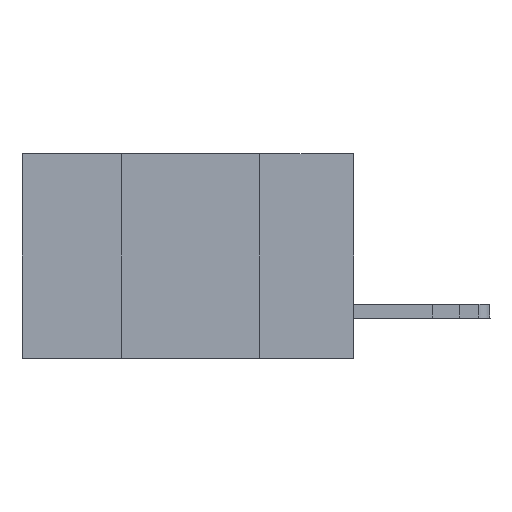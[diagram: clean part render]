
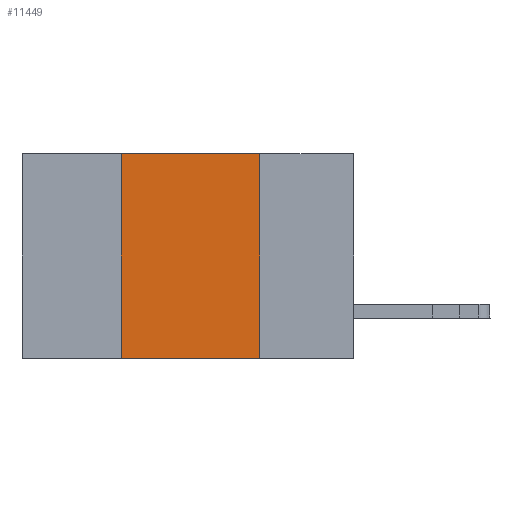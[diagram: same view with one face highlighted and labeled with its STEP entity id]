
A CAD part, left-side view. The second image highlights one B-rep face of the part: STEP entity #11449.
In plain terms, the highlighted planar face has unit normal (-1, 0, 0).
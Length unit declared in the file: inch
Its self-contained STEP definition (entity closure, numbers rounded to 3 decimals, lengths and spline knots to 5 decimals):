
#353 = CARTESIAN_POINT ( 'NONE',  ( 0., 0.42, 0. ) ) ;
#633 = ORIENTED_EDGE ( 'NONE', *, *, #11389, .F. ) ;
#1819 = ORIENTED_EDGE ( 'NONE', *, *, #3543, .F. ) ;
#2001 = VECTOR ( 'NONE', #17645, 39.37008 ) ;
#2810 = CARTESIAN_POINT ( 'NONE',  ( 0., 0.17, 0. ) ) ;
#3543 = EDGE_CURVE ( 'NONE', #6142, #19580, #6987, .T. ) ;
#4345 = ORIENTED_EDGE ( 'NONE', *, *, #11777, .T. ) ;
#4548 = DIRECTION ( 'NONE',  ( 0., -1., 0. ) ) ;
#4571 = EDGE_LOOP ( 'NONE', ( #10133, #633, #1819, #4345 ) ) ;
#5294 = CARTESIAN_POINT ( 'NONE',  ( 0., 0.6, -0.37 ) ) ;
#6142 = VERTEX_POINT ( 'NONE', #9474 ) ;
#6627 = DIRECTION ( 'NONE',  ( 1., 0., 0. ) ) ;
#6987 = LINE ( 'NONE', #353, #10831 ) ;
#8468 = CARTESIAN_POINT ( 'NONE',  ( 0., 0.42, 0. ) ) ;
#8620 = VECTOR ( 'NONE', #10720, 39.37008 ) ;
#9474 = CARTESIAN_POINT ( 'NONE',  ( 0., 0.42, -0.37 ) ) ;
#9942 = LINE ( 'NONE', #19896, #14551 ) ;
#10050 = VERTEX_POINT ( 'NONE', #18899 ) ;
#10133 = ORIENTED_EDGE ( 'NONE', *, *, #16684, .F. ) ;
#10710 = DIRECTION ( 'NONE',  ( 0., 0., 1. ) ) ;
#10720 = DIRECTION ( 'NONE',  ( 0., 0., -1. ) ) ;
#10831 = VECTOR ( 'NONE', #10710, 39.37008 ) ;
#11389 = EDGE_CURVE ( 'NONE', #19580, #10050, #9942, .T. ) ;
#11449 = ADVANCED_FACE ( 'NONE', ( #11870 ), #15551, .F. ) ;
#11777 = EDGE_CURVE ( 'NONE', #6142, #18393, #13797, .T. ) ;
#11870 = FACE_OUTER_BOUND ( 'NONE', #4571, .T. ) ;
#13797 = LINE ( 'NONE', #5294, #2001 ) ;
#14551 = VECTOR ( 'NONE', #4548, 39.37008 ) ;
#15406 = LINE ( 'NONE', #2810, #8620 ) ;
#15459 = AXIS2_PLACEMENT_3D ( 'NONE', #15886, #6627, #18944 ) ;
#15551 = PLANE ( 'NONE',  #15459 ) ;
#15886 = CARTESIAN_POINT ( 'NONE',  ( 0., 0.6, 0. ) ) ;
#16684 = EDGE_CURVE ( 'NONE', #10050, #18393, #15406, .T. ) ;
#17645 = DIRECTION ( 'NONE',  ( 0., -1., 0. ) ) ;
#18393 = VERTEX_POINT ( 'NONE', #19640 ) ;
#18899 = CARTESIAN_POINT ( 'NONE',  ( 0., 0.17, 0. ) ) ;
#18944 = DIRECTION ( 'NONE',  ( 0., 0., -1. ) ) ;
#19580 = VERTEX_POINT ( 'NONE', #8468 ) ;
#19640 = CARTESIAN_POINT ( 'NONE',  ( 0., 0.17, -0.37 ) ) ;
#19896 = CARTESIAN_POINT ( 'NONE',  ( 0., 0.6, 0. ) ) ;
